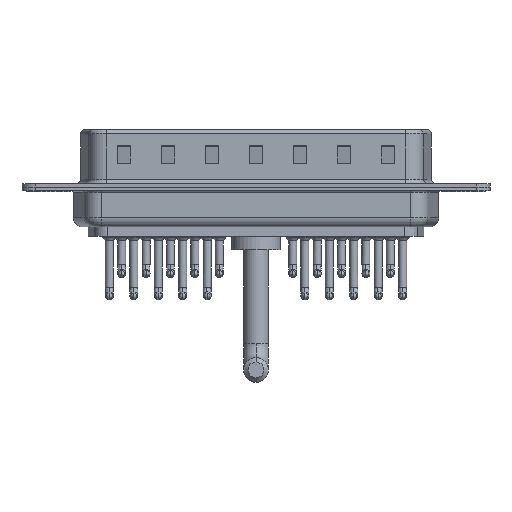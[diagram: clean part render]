
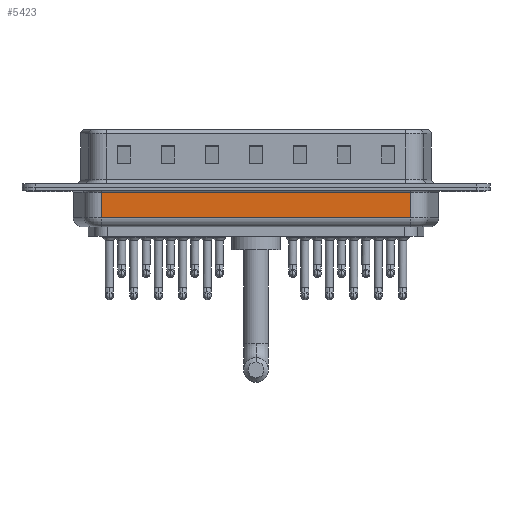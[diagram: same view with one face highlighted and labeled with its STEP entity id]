
A CAD part, front view. The second image highlights one B-rep face of the part: STEP entity #5423.
In plain terms, the highlighted planar face has unit normal (0, -1, 0).
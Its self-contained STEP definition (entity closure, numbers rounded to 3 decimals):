
#570 = FACE_OUTER_BOUND ( 'NONE', #3896, .T. ) ;
#656 = CARTESIAN_POINT ( 'NONE',  ( 6.006, -5.35, -0.65 ) ) ;
#770 = DIRECTION ( 'NONE',  ( -1., 0., 0. ) ) ;
#1109 = ORIENTED_EDGE ( 'NONE', *, *, #20994, .T. ) ;
#1843 = CARTESIAN_POINT ( 'NONE',  ( 6.006, -5.35, -4.5 ) ) ;
#3777 = LINE ( 'NONE', #1843, #19184 ) ;
#3896 = EDGE_LOOP ( 'NONE', ( #16390, #23568, #1109, #5422 ) ) ;
#4451 = CARTESIAN_POINT ( 'NONE',  ( 6.006, -5.35, -4.5 ) ) ;
#4498 = CARTESIAN_POINT ( 'NONE',  ( 41.044, -5.35, -0.65 ) ) ;
#4750 = AXIS2_PLACEMENT_3D ( 'NONE', #4451, #9960, #8139 ) ;
#5422 = ORIENTED_EDGE ( 'NONE', *, *, #18647, .T. ) ;
#5423 = ADVANCED_FACE ( 'NONE', ( #570 ), #8360, .F. ) ;
#6499 = LINE ( 'NONE', #19881, #21244 ) ;
#7425 = VERTEX_POINT ( 'NONE', #4498 ) ;
#8129 = CARTESIAN_POINT ( 'NONE',  ( 41.044, -5.35, -3.5 ) ) ;
#8139 = DIRECTION ( 'NONE',  ( 0., 0., 1. ) ) ;
#8360 = PLANE ( 'NONE',  #4750 ) ;
#9475 = LINE ( 'NONE', #17593, #21901 ) ;
#9960 = DIRECTION ( 'NONE',  ( 0., 1., 0. ) ) ;
#10729 = VERTEX_POINT ( 'NONE', #656 ) ;
#12067 = CARTESIAN_POINT ( 'NONE',  ( 6.006, -5.35, -3.5 ) ) ;
#13655 = CARTESIAN_POINT ( 'NONE',  ( 6.006, -5.35, -3.5 ) ) ;
#14026 = VERTEX_POINT ( 'NONE', #12067 ) ;
#16390 = ORIENTED_EDGE ( 'NONE', *, *, #22822, .F. ) ;
#17593 = CARTESIAN_POINT ( 'NONE',  ( 41.044, -5.35, -4.5 ) ) ;
#17941 = VERTEX_POINT ( 'NONE', #8129 ) ;
#18647 = EDGE_CURVE ( 'NONE', #7425, #10729, #6499, .T. ) ;
#19184 = VECTOR ( 'NONE', #22162, 1000. ) ;
#19223 = LINE ( 'NONE', #13655, #21117 ) ;
#19881 = CARTESIAN_POINT ( 'NONE',  ( 6.006, -5.35, -0.65 ) ) ;
#20420 = DIRECTION ( 'NONE',  ( 0., 0., 1. ) ) ;
#20994 = EDGE_CURVE ( 'NONE', #17941, #7425, #9475, .T. ) ;
#21117 = VECTOR ( 'NONE', #23109, 1000. ) ;
#21244 = VECTOR ( 'NONE', #770, 1000. ) ;
#21901 = VECTOR ( 'NONE', #20420, 1000. ) ;
#22162 = DIRECTION ( 'NONE',  ( 0., 0., 1. ) ) ;
#22822 = EDGE_CURVE ( 'NONE', #14026, #10729, #3777, .T. ) ;
#22894 = EDGE_CURVE ( 'NONE', #14026, #17941, #19223, .T. ) ;
#23109 = DIRECTION ( 'NONE',  ( 1., 0., 0. ) ) ;
#23568 = ORIENTED_EDGE ( 'NONE', *, *, #22894, .T. ) ;
